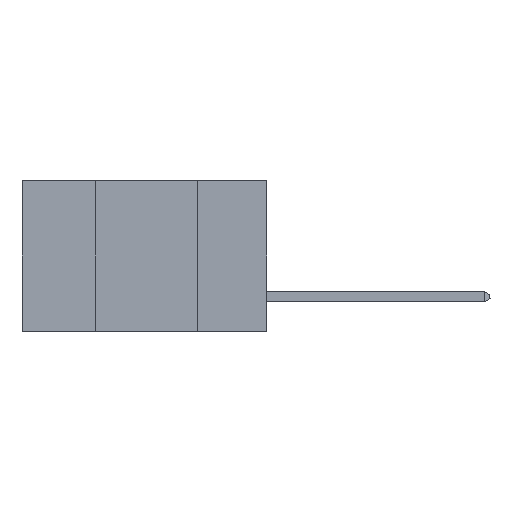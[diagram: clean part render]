
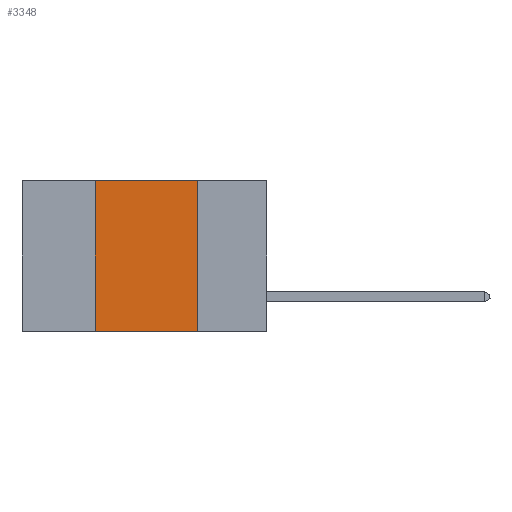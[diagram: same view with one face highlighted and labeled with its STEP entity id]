
A CAD part, left-side view. The second image highlights one B-rep face of the part: STEP entity #3348.
In plain terms, the highlighted planar face has unit normal (-1, 0, 0).
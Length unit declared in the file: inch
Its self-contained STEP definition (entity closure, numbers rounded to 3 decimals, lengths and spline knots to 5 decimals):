
#55 = VECTOR ( 'NONE', #1933, 39.37008 ) ;
#192 = VERTEX_POINT ( 'NONE', #5607 ) ;
#697 = EDGE_LOOP ( 'NONE', ( #1541, #6164, #8667, #7335 ) ) ;
#1302 = DIRECTION ( 'NONE',  ( 0., -1., 0. ) ) ;
#1541 = ORIENTED_EDGE ( 'NONE', *, *, #11008, .F. ) ;
#1933 = DIRECTION ( 'NONE',  ( 0., 0., -1. ) ) ;
#2021 = LINE ( 'NONE', #10538, #9652 ) ;
#2333 = DIRECTION ( 'NONE',  ( 0., 0., -1. ) ) ;
#2758 = FACE_OUTER_BOUND ( 'NONE', #697, .T. ) ;
#3348 = ADVANCED_FACE ( 'NONE', ( #2758 ), #12543, .F. ) ;
#3380 = DIRECTION ( 'NONE',  ( 1., 0., 0. ) ) ;
#3980 = LINE ( 'NONE', #6699, #11144 ) ;
#4792 = VERTEX_POINT ( 'NONE', #5207 ) ;
#5207 = CARTESIAN_POINT ( 'NONE',  ( 0., 0.17, 0. ) ) ;
#5607 = CARTESIAN_POINT ( 'NONE',  ( 0., 0.42, 0. ) ) ;
#6164 = ORIENTED_EDGE ( 'NONE', *, *, #6593, .F. ) ;
#6315 = CARTESIAN_POINT ( 'NONE',  ( 0., 0.6, 0. ) ) ;
#6593 = EDGE_CURVE ( 'NONE', #192, #4792, #10778, .T. ) ;
#6699 = CARTESIAN_POINT ( 'NONE',  ( 0., 0.42, 0. ) ) ;
#6784 = DIRECTION ( 'NONE',  ( 0., 0., 1. ) ) ;
#6821 = AXIS2_PLACEMENT_3D ( 'NONE', #6315, #3380, #2333 ) ;
#6901 = LINE ( 'NONE', #8615, #55 ) ;
#7335 = ORIENTED_EDGE ( 'NONE', *, *, #8925, .T. ) ;
#7436 = VECTOR ( 'NONE', #11060, 39.37008 ) ;
#8061 = VERTEX_POINT ( 'NONE', #12934 ) ;
#8615 = CARTESIAN_POINT ( 'NONE',  ( 0., 0.17, 0. ) ) ;
#8667 = ORIENTED_EDGE ( 'NONE', *, *, #12922, .F. ) ;
#8925 = EDGE_CURVE ( 'NONE', #10546, #8061, #2021, .T. ) ;
#9652 = VECTOR ( 'NONE', #1302, 39.37008 ) ;
#10216 = CARTESIAN_POINT ( 'NONE',  ( 0., 0.6, 0. ) ) ;
#10538 = CARTESIAN_POINT ( 'NONE',  ( 0., 0.6, -0.37 ) ) ;
#10546 = VERTEX_POINT ( 'NONE', #12966 ) ;
#10778 = LINE ( 'NONE', #10216, #7436 ) ;
#11008 = EDGE_CURVE ( 'NONE', #4792, #8061, #6901, .T. ) ;
#11060 = DIRECTION ( 'NONE',  ( 0., -1., 0. ) ) ;
#11144 = VECTOR ( 'NONE', #6784, 39.37008 ) ;
#12543 = PLANE ( 'NONE',  #6821 ) ;
#12922 = EDGE_CURVE ( 'NONE', #10546, #192, #3980, .T. ) ;
#12934 = CARTESIAN_POINT ( 'NONE',  ( 0., 0.17, -0.37 ) ) ;
#12966 = CARTESIAN_POINT ( 'NONE',  ( 0., 0.42, -0.37 ) ) ;
